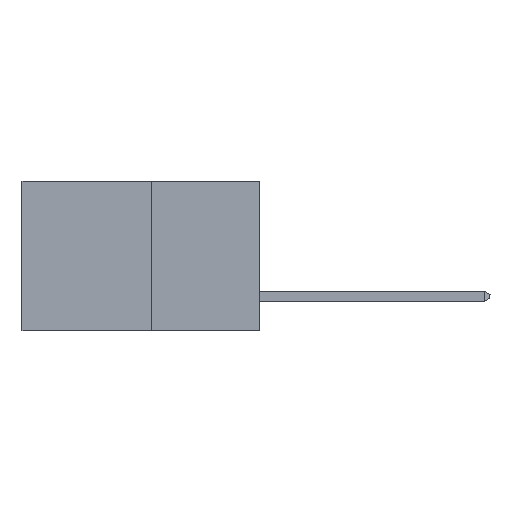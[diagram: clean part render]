
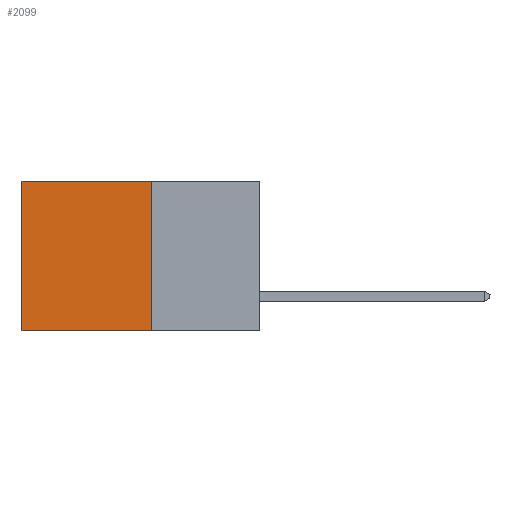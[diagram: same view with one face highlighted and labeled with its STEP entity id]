
A CAD part, left-side view. The second image highlights one B-rep face of the part: STEP entity #2099.
In plain terms, the highlighted planar face has unit normal (-1, 0, 0).
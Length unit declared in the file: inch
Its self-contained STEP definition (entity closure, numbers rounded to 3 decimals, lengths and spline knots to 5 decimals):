
#629 = EDGE_CURVE ( 'NONE', #10708, #726, #1200, .T. ) ;
#718 = CARTESIAN_POINT ( 'NONE',  ( 0.277, 0.27, -0.37 ) ) ;
#726 = VERTEX_POINT ( 'NONE', #718 ) ;
#830 = DIRECTION ( 'NONE',  ( 0., 0., -1. ) ) ;
#899 = VERTEX_POINT ( 'NONE', #12509 ) ;
#1030 = DIRECTION ( 'NONE',  ( 0., 1., 0. ) ) ;
#1138 = CARTESIAN_POINT ( 'NONE',  ( 0.277, 0.27, 0. ) ) ;
#1200 = LINE ( 'NONE', #7245, #9591 ) ;
#2099 = ADVANCED_FACE ( 'NONE', ( #8516 ), #12159, .F. ) ;
#2258 = DIRECTION ( 'NONE',  ( 0., 1., 0. ) ) ;
#2292 = VERTEX_POINT ( 'NONE', #14093 ) ;
#2680 = VECTOR ( 'NONE', #1030, 39.37008 ) ;
#3702 = AXIS2_PLACEMENT_3D ( 'NONE', #10342, #10791, #11887 ) ;
#3851 = VECTOR ( 'NONE', #2258, 39.37008 ) ;
#4009 = DIRECTION ( 'NONE',  ( 0., 0., -1. ) ) ;
#4101 = CARTESIAN_POINT ( 'NONE',  ( 0.277, 0.59, -0.37 ) ) ;
#4146 = LINE ( 'NONE', #4101, #11592 ) ;
#4557 = LINE ( 'NONE', #10187, #3851 ) ;
#6478 = EDGE_CURVE ( 'NONE', #10708, #2292, #11931, .T. ) ;
#6921 = EDGE_CURVE ( 'NONE', #2292, #899, #4146, .T. ) ;
#7245 = CARTESIAN_POINT ( 'NONE',  ( 0.277, 0.27, -0.37 ) ) ;
#8060 = ORIENTED_EDGE ( 'NONE', *, *, #6921, .T. ) ;
#8301 = ORIENTED_EDGE ( 'NONE', *, *, #13335, .F. ) ;
#8516 = FACE_OUTER_BOUND ( 'NONE', #10012, .T. ) ;
#8641 = ORIENTED_EDGE ( 'NONE', *, *, #629, .F. ) ;
#8657 = ORIENTED_EDGE ( 'NONE', *, *, #6478, .T. ) ;
#9591 = VECTOR ( 'NONE', #830, 39.37008 ) ;
#10012 = EDGE_LOOP ( 'NONE', ( #8060, #8301, #8641, #8657 ) ) ;
#10187 = CARTESIAN_POINT ( 'NONE',  ( 0.277, 0.27, -0.37 ) ) ;
#10342 = CARTESIAN_POINT ( 'NONE',  ( 0.277, 0.27, -0.37 ) ) ;
#10708 = VERTEX_POINT ( 'NONE', #12780 ) ;
#10791 = DIRECTION ( 'NONE',  ( 1., 0., 0. ) ) ;
#11592 = VECTOR ( 'NONE', #4009, 39.37008 ) ;
#11887 = DIRECTION ( 'NONE',  ( 0., 0., -1. ) ) ;
#11931 = LINE ( 'NONE', #1138, #2680 ) ;
#12159 = PLANE ( 'NONE',  #3702 ) ;
#12509 = CARTESIAN_POINT ( 'NONE',  ( 0.277, 0.59, -0.37 ) ) ;
#12780 = CARTESIAN_POINT ( 'NONE',  ( 0.277, 0.27, 0. ) ) ;
#13335 = EDGE_CURVE ( 'NONE', #726, #899, #4557, .T. ) ;
#14093 = CARTESIAN_POINT ( 'NONE',  ( 0.277, 0.59, 0. ) ) ;
